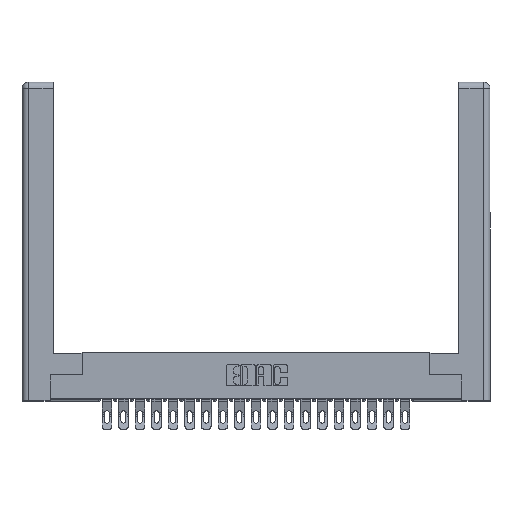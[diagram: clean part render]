
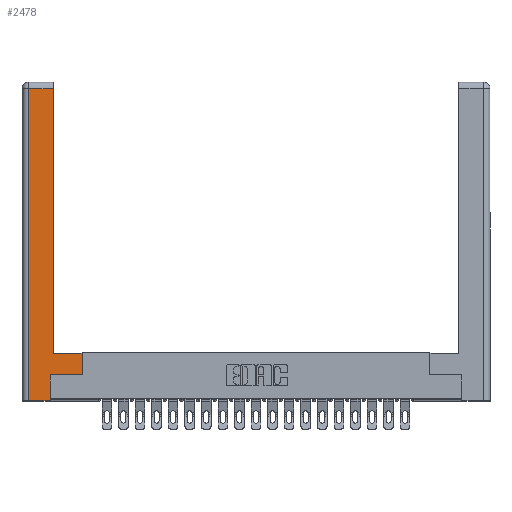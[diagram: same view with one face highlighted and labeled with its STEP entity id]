
A CAD part, top view. The second image highlights one B-rep face of the part: STEP entity #2478.
In plain terms, the highlighted planar face has unit normal (0, 0, 1).
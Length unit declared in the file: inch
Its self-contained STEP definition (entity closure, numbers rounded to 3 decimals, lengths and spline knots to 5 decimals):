
#427 = ORIENTED_EDGE ( 'NONE', *, *, #12707, .T. ) ;
#524 = VECTOR ( 'NONE', #5275, 39.37008 ) ;
#862 = CARTESIAN_POINT ( 'NONE',  ( 0.0615, 2.94, 0. ) ) ;
#1084 = PLANE ( 'NONE',  #20229 ) ;
#1207 = ORIENTED_EDGE ( 'NONE', *, *, #7975, .T. ) ;
#1611 = CARTESIAN_POINT ( 'NONE',  ( 0.265, 0.245, 0. ) ) ;
#1948 = DIRECTION ( 'NONE',  ( 0., -1., 0. ) ) ;
#1970 = DIRECTION ( 'NONE',  ( -1., 0., 0. ) ) ;
#2454 = EDGE_CURVE ( 'NONE', #15583, #12593, #10156, .T. ) ;
#2478 = ADVANCED_FACE ( 'NONE', ( #4974 ), #1084, .F. ) ;
#3296 = CARTESIAN_POINT ( 'NONE',  ( 0.565, 0.45, 0. ) ) ;
#3329 = VERTEX_POINT ( 'NONE', #11439 ) ;
#3799 = CARTESIAN_POINT ( 'NONE',  ( 0.0615, 0., 0. ) ) ;
#4864 = CARTESIAN_POINT ( 'NONE',  ( 0.295, 2.94, 0. ) ) ;
#4974 = FACE_OUTER_BOUND ( 'NONE', #18221, .T. ) ;
#5038 = CARTESIAN_POINT ( 'NONE',  ( 0.265, 0., 0. ) ) ;
#5269 = VECTOR ( 'NONE', #1970, 39.37008 ) ;
#5275 = DIRECTION ( 'NONE',  ( 0., 1., 0. ) ) ;
#5666 = ORIENTED_EDGE ( 'NONE', *, *, #17157, .T. ) ;
#7975 = EDGE_CURVE ( 'NONE', #19677, #25057, #13014, .T. ) ;
#8918 = EDGE_CURVE ( 'NONE', #12697, #19677, #19064, .T. ) ;
#9638 = ORIENTED_EDGE ( 'NONE', *, *, #2454, .T. ) ;
#9923 = VERTEX_POINT ( 'NONE', #862 ) ;
#10156 = LINE ( 'NONE', #22826, #14946 ) ;
#10459 = LINE ( 'NONE', #26406, #5269 ) ;
#10711 = DIRECTION ( 'NONE',  ( 0., 1., 0. ) ) ;
#11439 = CARTESIAN_POINT ( 'NONE',  ( 0.0615, 0., 0. ) ) ;
#11559 = DIRECTION ( 'NONE',  ( 0., 1., 0. ) ) ;
#11837 = VECTOR ( 'NONE', #11559, 39.37008 ) ;
#12593 = VERTEX_POINT ( 'NONE', #4864 ) ;
#12644 = CARTESIAN_POINT ( 'NONE',  ( 0.565, 0.45, 0. ) ) ;
#12697 = VERTEX_POINT ( 'NONE', #15644 ) ;
#12707 = EDGE_CURVE ( 'NONE', #17402, #12697, #13419, .T. ) ;
#12785 = LINE ( 'NONE', #3799, #19808 ) ;
#13014 = LINE ( 'NONE', #3296, #524 ) ;
#13277 = DIRECTION ( 'NONE',  ( -1., 0., 0. ) ) ;
#13419 = LINE ( 'NONE', #1611, #11837 ) ;
#13998 = EDGE_CURVE ( 'NONE', #9923, #3329, #12785, .T. ) ;
#14946 = VECTOR ( 'NONE', #10711, 39.37008 ) ;
#15583 = VERTEX_POINT ( 'NONE', #22397 ) ;
#15644 = CARTESIAN_POINT ( 'NONE',  ( 0.265, 0.245, 0. ) ) ;
#15868 = CARTESIAN_POINT ( 'NONE',  ( 0.265, 0., 0. ) ) ;
#16372 = DIRECTION ( 'NONE',  ( 1., 0., 0. ) ) ;
#16652 = ORIENTED_EDGE ( 'NONE', *, *, #13998, .T. ) ;
#16779 = EDGE_CURVE ( 'NONE', #25057, #15583, #22350, .T. ) ;
#17157 = EDGE_CURVE ( 'NONE', #3329, #17402, #23005, .T. ) ;
#17402 = VERTEX_POINT ( 'NONE', #15868 ) ;
#17569 = DIRECTION ( 'NONE',  ( 0., 0., -1. ) ) ;
#18221 = EDGE_LOOP ( 'NONE', ( #9638, #22022, #16652, #5666, #427, #23691, #1207, #18940 ) ) ;
#18940 = ORIENTED_EDGE ( 'NONE', *, *, #16779, .T. ) ;
#19064 = LINE ( 'NONE', #24765, #24201 ) ;
#19135 = VECTOR ( 'NONE', #24515, 39.37008 ) ;
#19677 = VERTEX_POINT ( 'NONE', #25905 ) ;
#19808 = VECTOR ( 'NONE', #1948, 39.37008 ) ;
#20229 = AXIS2_PLACEMENT_3D ( 'NONE', #21619, #17569, #13277 ) ;
#20434 = CARTESIAN_POINT ( 'NONE',  ( 0.295, 0.45, 0. ) ) ;
#21619 = CARTESIAN_POINT ( 'NONE',  ( 0., 0., 0. ) ) ;
#22022 = ORIENTED_EDGE ( 'NONE', *, *, #23048, .T. ) ;
#22350 = LINE ( 'NONE', #20434, #19135 ) ;
#22397 = CARTESIAN_POINT ( 'NONE',  ( 0.295, 0.45, 0. ) ) ;
#22826 = CARTESIAN_POINT ( 'NONE',  ( 0.295, 3., 0. ) ) ;
#23005 = LINE ( 'NONE', #5038, #25602 ) ;
#23048 = EDGE_CURVE ( 'NONE', #12593, #9923, #10459, .T. ) ;
#23691 = ORIENTED_EDGE ( 'NONE', *, *, #8918, .T. ) ;
#24201 = VECTOR ( 'NONE', #16372, 39.37008 ) ;
#24515 = DIRECTION ( 'NONE',  ( -1., 0., 0. ) ) ;
#24765 = CARTESIAN_POINT ( 'NONE',  ( 0.565, 0.245, 0. ) ) ;
#25057 = VERTEX_POINT ( 'NONE', #12644 ) ;
#25574 = DIRECTION ( 'NONE',  ( 1., 0., 0. ) ) ;
#25602 = VECTOR ( 'NONE', #25574, 39.37008 ) ;
#25905 = CARTESIAN_POINT ( 'NONE',  ( 0.565, 0.245, 0. ) ) ;
#26406 = CARTESIAN_POINT ( 'NONE',  ( 0.0615, 2.94, 0. ) ) ;
